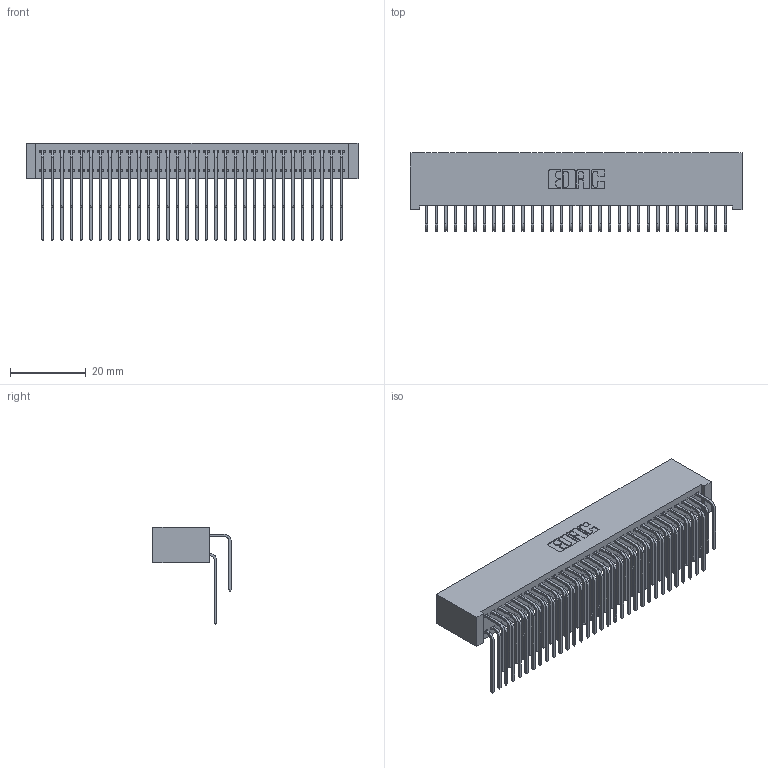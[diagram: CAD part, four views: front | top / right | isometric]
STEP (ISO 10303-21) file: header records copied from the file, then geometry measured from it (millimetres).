
FILE_DESCRIPTION (( 'STEP AP203' ), '1' );
FILE_NAME ('342-064-559-201.STEP', '2019-10-03T14:37:23', ( '' ), ( '' ), 'SwSTEP 2.0', 'SolidWorks 2016', '' );
FILE_SCHEMA (( 'CONFIG_CONTROL_DESIGN' ));
Length unit declared in the file: inch
Products named in the file (4): 345-292-001_558 559 Tail - 1; 345-292-001_559 Tail - 2; 342-064-559-201; 342 Part_Lugless
Assembly tree (65 placements, depth 2):
  342-064-559-201
    342 Part_Lugless
    345-292-001_558 559 Tail - 1  x32
    345-292-001_559 Tail - 2  x32
Bounding box: 87.53 x 20.64 x 25.78 mm (x, y, z)
Volume: 8625.8 mm3; surface area: 15910.6 mm2
Topology: 65 solids, 65 shells, 3558 faces, 10579 edges, 6966 vertices
Faces by surface type: plane 2494, cylinder 1064
Entity records: 23255 total; most frequent: CARTESIAN_POINT 3913, ORIENTED_EDGE 3798, DIRECTION 3335, EDGE_CURVE 1899, LINE 1739, VECTOR 1739, VERTEX_POINT 1262, AXIS2_PLACEMENT_3D 798
